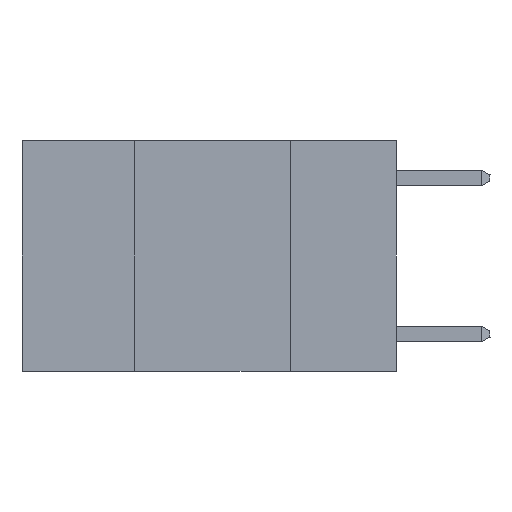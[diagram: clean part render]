
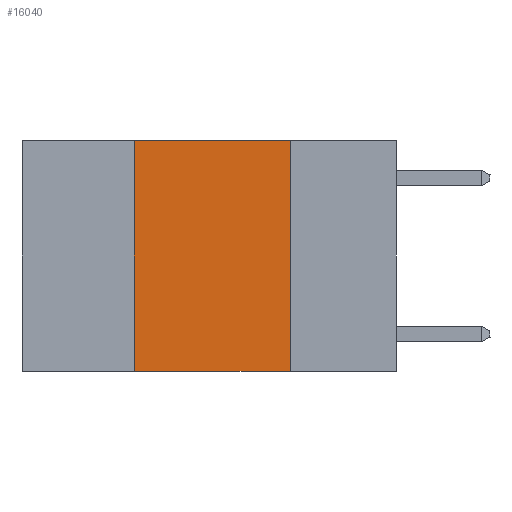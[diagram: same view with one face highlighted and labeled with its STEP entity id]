
A CAD part, left-side view. The second image highlights one B-rep face of the part: STEP entity #16040.
In plain terms, the highlighted planar face has unit normal (-1, 0, 0).
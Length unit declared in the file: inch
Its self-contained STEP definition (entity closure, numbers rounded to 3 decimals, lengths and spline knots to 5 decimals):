
#337 = ORIENTED_EDGE ( 'NONE', *, *, #9945, .T. ) ;
#578 = LINE ( 'NONE', #15067, #19036 ) ;
#715 = ORIENTED_EDGE ( 'NONE', *, *, #20353, .F. ) ;
#1462 = CARTESIAN_POINT ( 'NONE',  ( 0., 0.42, -0.37 ) ) ;
#1717 = PLANE ( 'NONE',  #7371 ) ;
#1875 = CARTESIAN_POINT ( 'NONE',  ( 0., 0.17, 0. ) ) ;
#3698 = EDGE_LOOP ( 'NONE', ( #6699, #6388, #715, #337 ) ) ;
#4580 = EDGE_CURVE ( 'NONE', #7037, #8811, #578, .T. ) ;
#5191 = VECTOR ( 'NONE', #5303, 39.37008 ) ;
#5303 = DIRECTION ( 'NONE',  ( 0., 0., 1. ) ) ;
#5478 = VERTEX_POINT ( 'NONE', #15597 ) ;
#6388 = ORIENTED_EDGE ( 'NONE', *, *, #11320, .F. ) ;
#6569 = LINE ( 'NONE', #8954, #10221 ) ;
#6699 = ORIENTED_EDGE ( 'NONE', *, *, #4580, .F. ) ;
#6889 = LINE ( 'NONE', #14938, #15602 ) ;
#7037 = VERTEX_POINT ( 'NONE', #1875 ) ;
#7371 = AXIS2_PLACEMENT_3D ( 'NONE', #23934, #9749, #20033 ) ;
#8346 = VERTEX_POINT ( 'NONE', #1462 ) ;
#8811 = VERTEX_POINT ( 'NONE', #17808 ) ;
#8954 = CARTESIAN_POINT ( 'NONE',  ( 0., 0.6, 0. ) ) ;
#9749 = DIRECTION ( 'NONE',  ( 1., 0., 0. ) ) ;
#9776 = DIRECTION ( 'NONE',  ( 0., -1., 0. ) ) ;
#9945 = EDGE_CURVE ( 'NONE', #8346, #8811, #6889, .T. ) ;
#10221 = VECTOR ( 'NONE', #12782, 39.37008 ) ;
#11320 = EDGE_CURVE ( 'NONE', #5478, #7037, #6569, .T. ) ;
#12782 = DIRECTION ( 'NONE',  ( 0., -1., 0. ) ) ;
#14938 = CARTESIAN_POINT ( 'NONE',  ( 0., 0.6, -0.37 ) ) ;
#15067 = CARTESIAN_POINT ( 'NONE',  ( 0., 0.17, 0. ) ) ;
#15597 = CARTESIAN_POINT ( 'NONE',  ( 0., 0.42, 0. ) ) ;
#15602 = VECTOR ( 'NONE', #9776, 39.37008 ) ;
#16040 = ADVANCED_FACE ( 'NONE', ( #18049 ), #1717, .F. ) ;
#16839 = LINE ( 'NONE', #22732, #5191 ) ;
#17808 = CARTESIAN_POINT ( 'NONE',  ( 0., 0.17, -0.37 ) ) ;
#18049 = FACE_OUTER_BOUND ( 'NONE', #3698, .T. ) ;
#19036 = VECTOR ( 'NONE', #24762, 39.37008 ) ;
#20033 = DIRECTION ( 'NONE',  ( 0., 0., -1. ) ) ;
#20353 = EDGE_CURVE ( 'NONE', #8346, #5478, #16839, .T. ) ;
#22732 = CARTESIAN_POINT ( 'NONE',  ( 0., 0.42, 0. ) ) ;
#23934 = CARTESIAN_POINT ( 'NONE',  ( 0., 0.6, 0. ) ) ;
#24762 = DIRECTION ( 'NONE',  ( 0., 0., -1. ) ) ;
